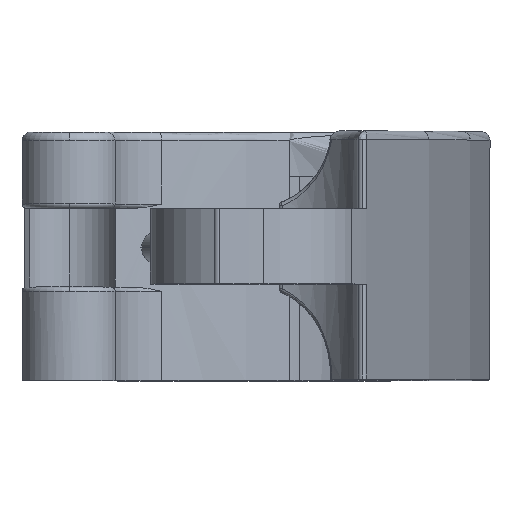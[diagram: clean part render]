
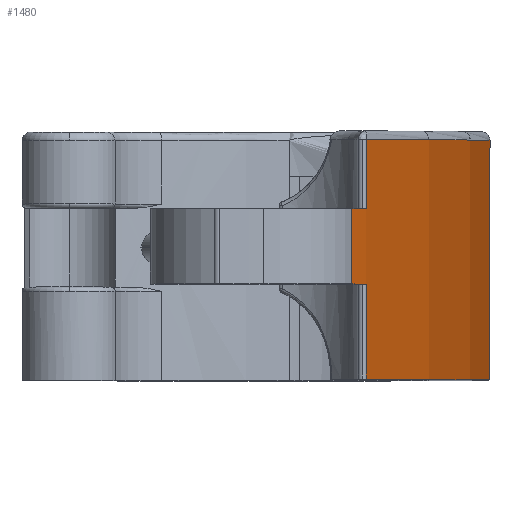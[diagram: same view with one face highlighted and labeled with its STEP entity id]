
A CAD part, top view. The second image highlights one B-rep face of the part: STEP entity #1480.
In plain terms, the highlighted cylindrical face has radius 180.483 mm (diameter 360.965 mm), a partial arc.
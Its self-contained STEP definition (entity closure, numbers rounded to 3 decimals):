
#12 = VECTOR ( 'NONE', #451, 1000. ) ;
#277 = CARTESIAN_POINT ( 'NONE',  ( -5.58, 10.6, 126.359 ) ) ;
#286 = EDGE_CURVE ( 'NONE', #458, #2404, #1649, .T. ) ;
#294 = AXIS2_PLACEMENT_3D ( 'NONE', #1950, #2470, #1065 ) ;
#397 = ORIENTED_EDGE ( 'NONE', *, *, #4565, .F. ) ;
#451 = DIRECTION ( 'NONE',  ( 0., 1., 0. ) ) ;
#458 = VERTEX_POINT ( 'NONE', #5396 ) ;
#569 = EDGE_CURVE ( 'NONE', #2028, #1953, #3080, .T. ) ;
#579 = ORIENTED_EDGE ( 'NONE', *, *, #569, .T. ) ;
#703 = VECTOR ( 'NONE', #1250, 1000. ) ;
#715 = VERTEX_POINT ( 'NONE', #5470 ) ;
#732 = CARTESIAN_POINT ( 'NONE',  ( -3.859, 1.5, 122.48 ) ) ;
#742 = ORIENTED_EDGE ( 'NONE', *, *, #3285, .T. ) ;
#780 = EDGE_CURVE ( 'NONE', #2160, #715, #3467, .T. ) ;
#789 = LINE ( 'NONE', #1701, #703 ) ;
#806 = DIRECTION ( 'NONE',  ( 0., 1., 0. ) ) ;
#821 = DIRECTION ( 'NONE',  ( 0., 0., 1. ) ) ;
#840 = AXIS2_PLACEMENT_3D ( 'NONE', #3518, #2608, #2576 ) ;
#879 = CARTESIAN_POINT ( 'NONE',  ( -169.67, 1.5, 51.202 ) ) ;
#1065 = DIRECTION ( 'NONE',  ( 0., 0., 1. ) ) ;
#1226 = LINE ( 'NONE', #3540, #5829 ) ;
#1250 = DIRECTION ( 'NONE',  ( 0., -1., 0. ) ) ;
#1298 = FACE_OUTER_BOUND ( 'NONE', #3411, .T. ) ;
#1410 = CARTESIAN_POINT ( 'NONE',  ( -3.859, -0.5, 122.48 ) ) ;
#1480 = ADVANCED_FACE ( 'NONE', ( #1298 ), #5583, .T. ) ;
#1505 = ORIENTED_EDGE ( 'NONE', *, *, #780, .T. ) ;
#1525 = CIRCLE ( 'NONE', #5730, 180.483 ) ;
#1649 = CIRCLE ( 'NONE', #294, 180.483 ) ;
#1701 = CARTESIAN_POINT ( 'NONE',  ( -3.859, 1.5, 122.48 ) ) ;
#1793 = ORIENTED_EDGE ( 'NONE', *, *, #5782, .T. ) ;
#1828 = EDGE_CURVE ( 'NONE', #3902, #2028, #1226, .T. ) ;
#1950 = CARTESIAN_POINT ( 'NONE',  ( -169.67, 27.5, 51.202 ) ) ;
#1953 = VERTEX_POINT ( 'NONE', #4524 ) ;
#2005 = AXIS2_PLACEMENT_3D ( 'NONE', #3081, #2139, #821 ) ;
#2028 = VERTEX_POINT ( 'NONE', #277 ) ;
#2121 = ORIENTED_EDGE ( 'NONE', *, *, #286, .T. ) ;
#2139 = DIRECTION ( 'NONE',  ( 0., 1., 0. ) ) ;
#2160 = VERTEX_POINT ( 'NONE', #1410 ) ;
#2404 = VERTEX_POINT ( 'NONE', #2925 ) ;
#2418 = VERTEX_POINT ( 'NONE', #5743 ) ;
#2470 = DIRECTION ( 'NONE',  ( 0., -1., 0. ) ) ;
#2576 = DIRECTION ( 'NONE',  ( 0., 0., -1. ) ) ;
#2608 = DIRECTION ( 'NONE',  ( 0., 1., 0. ) ) ;
#2665 = DIRECTION ( 'NONE',  ( 0., 0., 1. ) ) ;
#2796 = DIRECTION ( 'NONE',  ( 0., 0., -1. ) ) ;
#2925 = CARTESIAN_POINT ( 'NONE',  ( -3.859, 27.5, 122.48 ) ) ;
#3080 = CIRCLE ( 'NONE', #2005, 180.483 ) ;
#3081 = CARTESIAN_POINT ( 'NONE',  ( -169.67, 10.6, 51.202 ) ) ;
#3130 = ORIENTED_EDGE ( 'NONE', *, *, #1828, .T. ) ;
#3235 = CARTESIAN_POINT ( 'NONE',  ( -5.58, 19.4, 126.359 ) ) ;
#3285 = EDGE_CURVE ( 'NONE', #2404, #2418, #4919, .T. ) ;
#3291 = CARTESIAN_POINT ( 'NONE',  ( 2.267, 1.5, -3.677 ) ) ;
#3411 = EDGE_LOOP ( 'NONE', ( #579, #3431, #1505, #1793, #2121, #742, #397, #3130 ) ) ;
#3431 = ORIENTED_EDGE ( 'NONE', *, *, #5664, .T. ) ;
#3467 = CIRCLE ( 'NONE', #840, 180.483 ) ;
#3512 = DIRECTION ( 'NONE',  ( 0., -1., 0. ) ) ;
#3518 = CARTESIAN_POINT ( 'NONE',  ( -169.67, -0.5, 51.202 ) ) ;
#3540 = CARTESIAN_POINT ( 'NONE',  ( -5.58, 1.5, 126.359 ) ) ;
#3902 = VERTEX_POINT ( 'NONE', #3235 ) ;
#4006 = DIRECTION ( 'NONE',  ( 0., -1., 0. ) ) ;
#4245 = LINE ( 'NONE', #3291, #12 ) ;
#4250 = VECTOR ( 'NONE', #3512, 1000. ) ;
#4524 = CARTESIAN_POINT ( 'NONE',  ( -3.859, 10.6, 122.48 ) ) ;
#4565 = EDGE_CURVE ( 'NONE', #3902, #2418, #1525, .T. ) ;
#4919 = LINE ( 'NONE', #732, #4250 ) ;
#4993 = CARTESIAN_POINT ( 'NONE',  ( -169.67, 19.4, 51.202 ) ) ;
#5396 = CARTESIAN_POINT ( 'NONE',  ( 2.267, 27.5, -3.677 ) ) ;
#5470 = CARTESIAN_POINT ( 'NONE',  ( 2.267, -0.5, -3.677 ) ) ;
#5583 = CYLINDRICAL_SURFACE ( 'NONE', #5656, 180.483 ) ;
#5656 = AXIS2_PLACEMENT_3D ( 'NONE', #879, #6041, #2796 ) ;
#5664 = EDGE_CURVE ( 'NONE', #1953, #2160, #789, .T. ) ;
#5730 = AXIS2_PLACEMENT_3D ( 'NONE', #4993, #806, #2665 ) ;
#5743 = CARTESIAN_POINT ( 'NONE',  ( -3.859, 19.4, 122.48 ) ) ;
#5782 = EDGE_CURVE ( 'NONE', #715, #458, #4245, .T. ) ;
#5829 = VECTOR ( 'NONE', #4006, 1000. ) ;
#6041 = DIRECTION ( 'NONE',  ( 0., -1., 0. ) ) ;
